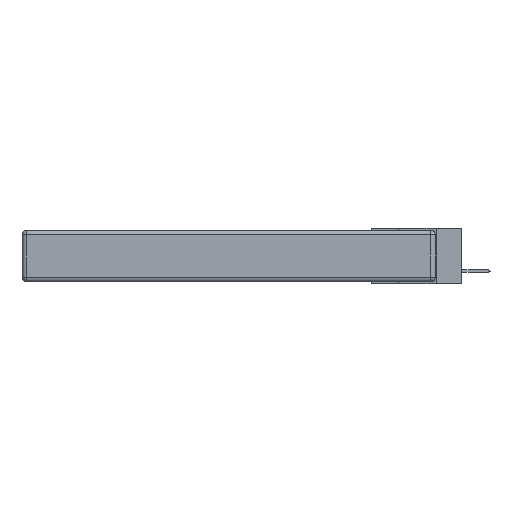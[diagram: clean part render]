
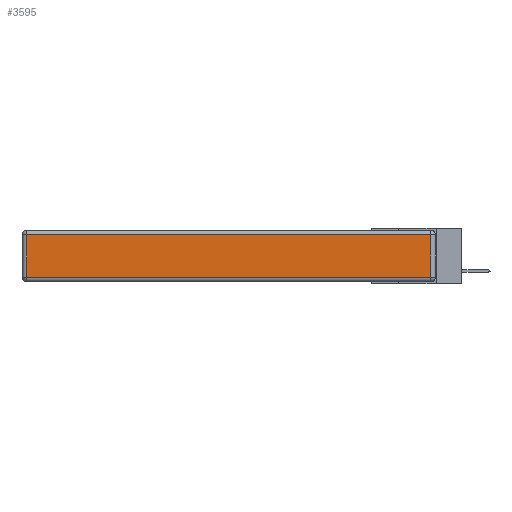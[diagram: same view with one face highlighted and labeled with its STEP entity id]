
A CAD part, left-side view. The second image highlights one B-rep face of the part: STEP entity #3595.
In plain terms, the highlighted planar face has unit normal (-1, 0, 0).
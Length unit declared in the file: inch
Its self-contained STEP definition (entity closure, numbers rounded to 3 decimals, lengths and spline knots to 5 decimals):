
#1647 = DIRECTION ( 'NONE',  ( 0., 1., 0. ) ) ;
#1689 = LINE ( 'NONE', #11973, #6305 ) ;
#1720 = CARTESIAN_POINT ( 'NONE',  ( 0., 0.03, -0.03 ) ) ;
#2213 = DIRECTION ( 'NONE',  ( 0., 0., 1. ) ) ;
#2669 = EDGE_CURVE ( 'NONE', #10898, #14041, #11416, .T. ) ;
#3388 = EDGE_LOOP ( 'NONE', ( #14669, #5446, #15780, #3497 ) ) ;
#3497 = ORIENTED_EDGE ( 'NONE', *, *, #2669, .T. ) ;
#3595 = ADVANCED_FACE ( 'NONE', ( #17012 ), #10934, .T. ) ;
#3613 = CARTESIAN_POINT ( 'NONE',  ( 0., 0.03, -0.343 ) ) ;
#3799 = DIRECTION ( 'NONE',  ( 0., 0., 1. ) ) ;
#4458 = CARTESIAN_POINT ( 'NONE',  ( 0., 2.72, -0.313 ) ) ;
#5446 = ORIENTED_EDGE ( 'NONE', *, *, #6921, .T. ) ;
#5669 = EDGE_CURVE ( 'NONE', #14041, #6043, #1689, .T. ) ;
#5702 = CARTESIAN_POINT ( 'NONE',  ( 0., 0., -0.343 ) ) ;
#5762 = DIRECTION ( 'NONE',  ( -1., 0., 0. ) ) ;
#5911 = VECTOR ( 'NONE', #9512, 39.37008 ) ;
#6043 = VERTEX_POINT ( 'NONE', #11044 ) ;
#6305 = VECTOR ( 'NONE', #6735, 39.37008 ) ;
#6735 = DIRECTION ( 'NONE',  ( 0., -1., 0. ) ) ;
#6921 = EDGE_CURVE ( 'NONE', #6043, #13233, #16257, .T. ) ;
#8981 = LINE ( 'NONE', #13352, #16106 ) ;
#9512 = DIRECTION ( 'NONE',  ( 0., 0., -1. ) ) ;
#10140 = AXIS2_PLACEMENT_3D ( 'NONE', #5702, #5762, #3799 ) ;
#10898 = VERTEX_POINT ( 'NONE', #16349 ) ;
#10934 = PLANE ( 'NONE',  #10140 ) ;
#11044 = CARTESIAN_POINT ( 'NONE',  ( 0., 0.03, -0.313 ) ) ;
#11416 = LINE ( 'NONE', #14987, #5911 ) ;
#11973 = CARTESIAN_POINT ( 'NONE',  ( 0., 0., -0.313 ) ) ;
#13233 = VERTEX_POINT ( 'NONE', #1720 ) ;
#13352 = CARTESIAN_POINT ( 'NONE',  ( 0., 2.75, -0.03 ) ) ;
#14041 = VERTEX_POINT ( 'NONE', #4458 ) ;
#14669 = ORIENTED_EDGE ( 'NONE', *, *, #5669, .T. ) ;
#14987 = CARTESIAN_POINT ( 'NONE',  ( 0., 2.72, -0.343 ) ) ;
#15033 = VECTOR ( 'NONE', #2213, 39.37008 ) ;
#15780 = ORIENTED_EDGE ( 'NONE', *, *, #16643, .T. ) ;
#16106 = VECTOR ( 'NONE', #1647, 39.37008 ) ;
#16257 = LINE ( 'NONE', #3613, #15033 ) ;
#16349 = CARTESIAN_POINT ( 'NONE',  ( 0., 2.72, -0.03 ) ) ;
#16643 = EDGE_CURVE ( 'NONE', #13233, #10898, #8981, .T. ) ;
#17012 = FACE_OUTER_BOUND ( 'NONE', #3388, .T. ) ;
